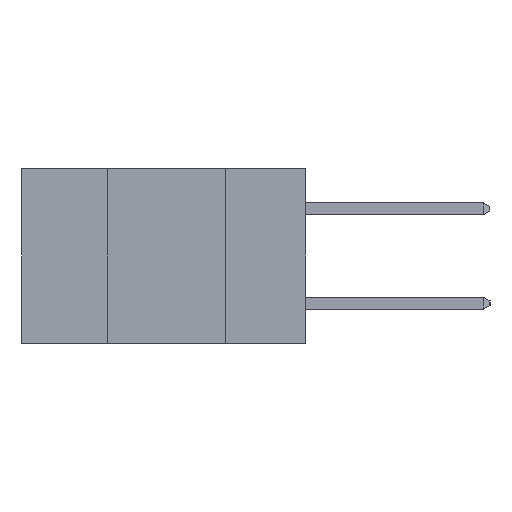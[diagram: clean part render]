
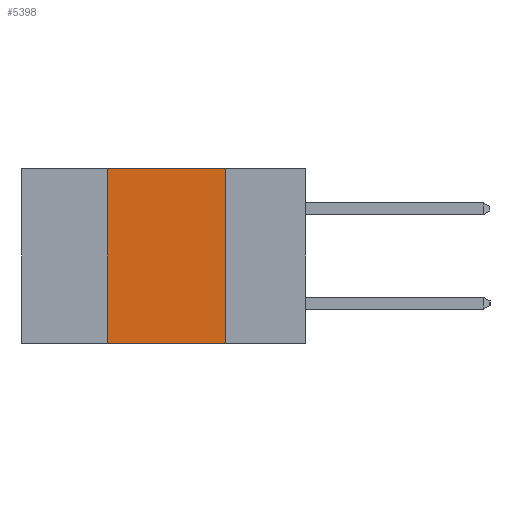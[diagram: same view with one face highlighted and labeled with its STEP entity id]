
A CAD part, left-side view. The second image highlights one B-rep face of the part: STEP entity #5398.
In plain terms, the highlighted planar face has unit normal (-1, 0, 0).
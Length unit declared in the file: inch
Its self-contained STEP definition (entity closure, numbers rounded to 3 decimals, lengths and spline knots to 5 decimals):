
#450 = EDGE_CURVE ( 'NONE', #2676, #4352, #5630, .T. ) ;
#703 = VECTOR ( 'NONE', #9921, 39.37008 ) ;
#714 = VECTOR ( 'NONE', #3562, 39.37008 ) ;
#909 = EDGE_CURVE ( 'NONE', #8200, #4352, #10856, .T. ) ;
#1420 = AXIS2_PLACEMENT_3D ( 'NONE', #2054, #2965, #9531 ) ;
#1725 = ORIENTED_EDGE ( 'NONE', *, *, #9410, .F. ) ;
#2037 = DIRECTION ( 'NONE',  ( 0., -1., 0. ) ) ;
#2054 = CARTESIAN_POINT ( 'NONE',  ( 0., 0.6, 0. ) ) ;
#2634 = CARTESIAN_POINT ( 'NONE',  ( 0., 0.6, -0.37 ) ) ;
#2676 = VERTEX_POINT ( 'NONE', #7970 ) ;
#2838 = ORIENTED_EDGE ( 'NONE', *, *, #3111, .F. ) ;
#2965 = DIRECTION ( 'NONE',  ( 1., 0., 0. ) ) ;
#3111 = EDGE_CURVE ( 'NONE', #4030, #8200, #7242, .T. ) ;
#3562 = DIRECTION ( 'NONE',  ( 0., -1., 0. ) ) ;
#3744 = CARTESIAN_POINT ( 'NONE',  ( 0., 0.17, -0.37 ) ) ;
#4018 = EDGE_LOOP ( 'NONE', ( #5593, #2838, #1725, #4317 ) ) ;
#4030 = VERTEX_POINT ( 'NONE', #4208 ) ;
#4208 = CARTESIAN_POINT ( 'NONE',  ( 0., 0.42, 0. ) ) ;
#4317 = ORIENTED_EDGE ( 'NONE', *, *, #450, .T. ) ;
#4352 = VERTEX_POINT ( 'NONE', #3744 ) ;
#5398 = ADVANCED_FACE ( 'NONE', ( #7642 ), #7673, .F. ) ;
#5593 = ORIENTED_EDGE ( 'NONE', *, *, #909, .F. ) ;
#5630 = LINE ( 'NONE', #2634, #714 ) ;
#6640 = VECTOR ( 'NONE', #2037, 39.37008 ) ;
#7242 = LINE ( 'NONE', #9513, #6640 ) ;
#7348 = CARTESIAN_POINT ( 'NONE',  ( 0., 0.42, -0.37 ) ) ;
#7390 = DIRECTION ( 'NONE',  ( 0., 0., 1. ) ) ;
#7642 = FACE_OUTER_BOUND ( 'NONE', #4018, .T. ) ;
#7673 = PLANE ( 'NONE',  #1420 ) ;
#7970 = CARTESIAN_POINT ( 'NONE',  ( 0., 0.42, -0.37 ) ) ;
#8200 = VERTEX_POINT ( 'NONE', #9443 ) ;
#9410 = EDGE_CURVE ( 'NONE', #2676, #4030, #9702, .T. ) ;
#9443 = CARTESIAN_POINT ( 'NONE',  ( 0., 0.17, 0. ) ) ;
#9513 = CARTESIAN_POINT ( 'NONE',  ( 0., 0.6, 0. ) ) ;
#9531 = DIRECTION ( 'NONE',  ( 0., 0., -1. ) ) ;
#9702 = LINE ( 'NONE', #7348, #11789 ) ;
#9921 = DIRECTION ( 'NONE',  ( 0., 0., -1. ) ) ;
#9969 = CARTESIAN_POINT ( 'NONE',  ( 0., 0.17, -0.37 ) ) ;
#10856 = LINE ( 'NONE', #9969, #703 ) ;
#11789 = VECTOR ( 'NONE', #7390, 39.37008 ) ;
